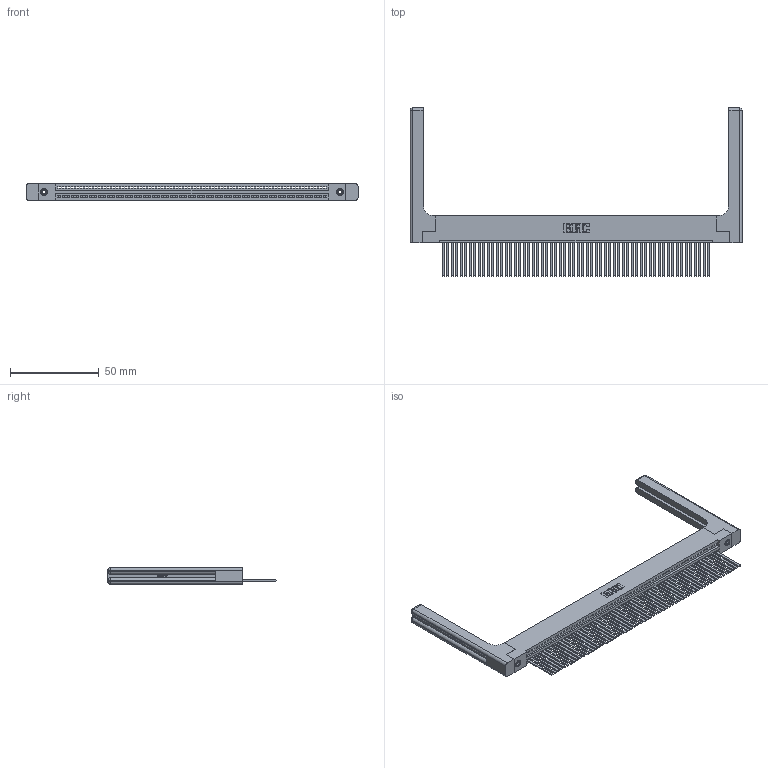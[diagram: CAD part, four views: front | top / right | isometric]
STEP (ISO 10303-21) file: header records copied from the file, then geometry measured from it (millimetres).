
FILE_DESCRIPTION (( 'STEP AP203' ), '1' );
FILE_NAME ('395-060-544-158.STEP', '2019-10-24T13:00:09', ( '' ), ( '' ), 'SwSTEP 2.0', 'SolidWorks 2016', '' );
FILE_SCHEMA (( 'CONFIG_CONTROL_DESIGN' ));
Length unit declared in the file: inch
Products named in the file (5): 345-220-058_345-220-058; 345-292-001_345-293-144; 345 Part_Flush Mounting Lugs - 0.156 Dia-TH; 345-250-001_345-250-001-102; 395-060-544-158
Assembly tree (65 placements, depth 2):
  395-060-544-158
    345 Part_Flush Mounting Lugs - 0.156 Dia-TH
    345-292-001_345-293-144  x60
    345-250-001_345-250-001-102  x2
    345-220-058_345-220-058  x2
Bounding box: 187.43 x 94.92 x 9.4 mm (x, y, z)
Volume: 27149.3 mm3; surface area: 32412.9 mm2
Topology: 65 solids, 65 shells, 3502 faces, 10487 edges, 6890 vertices
Faces by surface type: plane 2388, cylinder 1054, bspline 36, cone 12, sphere 8, torus 4
Entity records: 47732 total; most frequent: CARTESIAN_POINT 9237, ORIENTED_EDGE 8028, DIRECTION 6986, EDGE_CURVE 4014, VECTOR 3554, LINE 3554, VERTEX_POINT 2666, AXIS2_PLACEMENT_3D 1716
